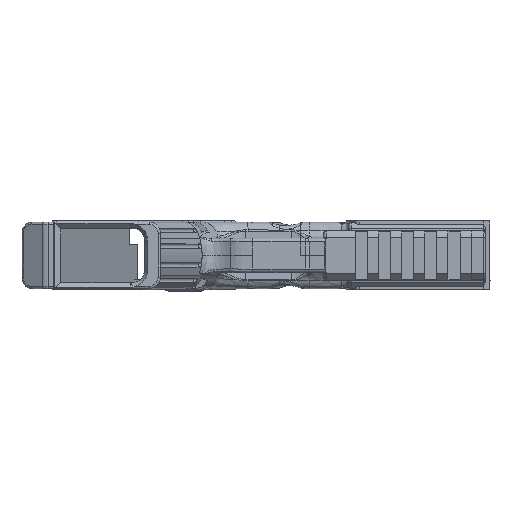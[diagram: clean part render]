
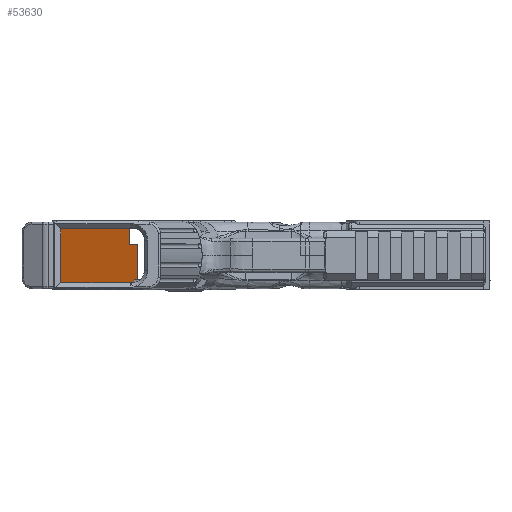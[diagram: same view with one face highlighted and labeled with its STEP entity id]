
A CAD part, front view. The second image highlights one B-rep face of the part: STEP entity #53630.
In plain terms, the highlighted planar face has unit normal (0.951, -0.309, 0).
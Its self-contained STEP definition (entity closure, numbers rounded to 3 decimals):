
#6615=FACE_OUTER_BOUND('',#9681,.T.);
#9681=EDGE_LOOP('',(#38541,#38542,#38543,#38544,#38545,#38546,#38547,#38548,
#38549,#38550));
#12887=LINE('',#80048,#17347);
#12902=LINE('',#80396,#17362);
#12956=LINE('',#83329,#17416);
#12957=LINE('',#83514,#17417);
#12977=LINE('',#83908,#17437);
#13246=LINE('',#92674,#17706);
#13247=LINE('',#92676,#17707);
#13248=LINE('',#92677,#17708);
#13249=LINE('',#92679,#17709);
#13250=LINE('',#92680,#17710);
#17347=VECTOR('',#59972,10.);
#17362=VECTOR('',#59995,10.);
#17416=VECTOR('',#60157,10.);
#17417=VECTOR('',#60166,10.);
#17437=VECTOR('',#60236,10.);
#17706=VECTOR('',#61247,10.);
#17707=VECTOR('',#61248,10.);
#17708=VECTOR('',#61249,10.);
#17709=VECTOR('',#61250,10.);
#17710=VECTOR('',#61251,10.);
#21906=VERTEX_POINT('',#80045);
#21907=VERTEX_POINT('',#80047);
#21927=VERTEX_POINT('',#80393);
#21928=VERTEX_POINT('',#80395);
#22034=VERTEX_POINT('',#83513);
#22059=VERTEX_POINT('',#83906);
#22441=VERTEX_POINT('',#92672);
#22442=VERTEX_POINT('',#92673);
#22443=VERTEX_POINT('',#92675);
#22444=VERTEX_POINT('',#92678);
#27706=EDGE_CURVE('',#21906,#21907,#12887,.T.);
#27731=EDGE_CURVE('',#21927,#21928,#12902,.T.);
#27868=EDGE_CURVE('',#21907,#21927,#12956,.T.);
#27874=EDGE_CURVE('',#21928,#22034,#12957,.T.);
#27911=EDGE_CURVE('',#22034,#22059,#12977,.T.);
#28570=EDGE_CURVE('',#22441,#22442,#13246,.T.);
#28571=EDGE_CURVE('',#22443,#22441,#13247,.F.);
#28572=EDGE_CURVE('',#22443,#22059,#13248,.T.);
#28573=EDGE_CURVE('',#21906,#22444,#13249,.T.);
#28574=EDGE_CURVE('',#22442,#22444,#13250,.F.);
#38541=ORIENTED_EDGE('',*,*,#28570,.F.);
#38542=ORIENTED_EDGE('',*,*,#28571,.F.);
#38543=ORIENTED_EDGE('',*,*,#28572,.T.);
#38544=ORIENTED_EDGE('',*,*,#27911,.F.);
#38545=ORIENTED_EDGE('',*,*,#27874,.F.);
#38546=ORIENTED_EDGE('',*,*,#27731,.F.);
#38547=ORIENTED_EDGE('',*,*,#27868,.F.);
#38548=ORIENTED_EDGE('',*,*,#27706,.F.);
#38549=ORIENTED_EDGE('',*,*,#28573,.T.);
#38550=ORIENTED_EDGE('',*,*,#28574,.F.);
#52053=PLANE('',#56979);
#53630=ADVANCED_FACE('',(#6615),#52053,.F.);
#56979=AXIS2_PLACEMENT_3D('',#92671,#61245,#61246);
#59972=DIRECTION('',(0.,0.,-1.));
#59995=DIRECTION('',(0.,0.,-1.));
#60157=DIRECTION('',(0.309,0.951,0.));
#60166=DIRECTION('',(-0.309,-0.951,0.));
#60236=DIRECTION('',(0.,0.,-1.));
#61245=DIRECTION('center_axis',(-0.951,0.309,0.));
#61246=DIRECTION('ref_axis',(0.,0.,
1.));
#61247=DIRECTION('',(0.,0.,1.));
#61248=DIRECTION('',(0.224,0.689,0.689));
#61249=DIRECTION('',(0.309,0.951,0.));
#61250=DIRECTION('',(-0.309,-0.951,0.));
#61251=DIRECTION('',(-0.224,-0.689,0.689));
#80045=CARTESIAN_POINT('',(30.049,-12.4,11.75));
#80047=CARTESIAN_POINT('',(30.049,-12.4,4.75));
#80048=CARTESIAN_POINT('',(30.049,-12.4,2.982));
#80393=CARTESIAN_POINT('',(33.591,-1.5,4.75));
#80395=CARTESIAN_POINT('',(33.591,-1.5,-10.375));
#80396=CARTESIAN_POINT('',(33.591,-1.5,-5.875));
#83329=CARTESIAN_POINT('',(18.86,-46.836,4.75));
#83513=CARTESIAN_POINT('',(32.169,-5.875,-10.375));
#83514=CARTESIAN_POINT('',(17.241,-51.82,-10.375));
#83906=CARTESIAN_POINT('',(32.169,-5.875,-11.75));
#83908=CARTESIAN_POINT('',(32.169,-5.875,-5.875));
#92671=CARTESIAN_POINT('Origin',(2.312,-97.765,-11.75));
#92672=CARTESIAN_POINT('',(0.579,-103.098,-11.848));
#92673=CARTESIAN_POINT('',(0.579,-103.098,11.848));
#92674=CARTESIAN_POINT('',(0.579,-103.098,-13.075));
#92675=CARTESIAN_POINT('',(0.611,-103.,-11.75));
#92676=CARTESIAN_POINT('',(0.788,-102.456,-11.206));
#92677=CARTESIAN_POINT('',(2.312,-97.765,-11.75));
#92678=CARTESIAN_POINT('',(0.611,-103.,11.75));
#92679=CARTESIAN_POINT('',(2.312,-97.765,11.75));
#92680=CARTESIAN_POINT('',(2.601,-96.876,5.626));
